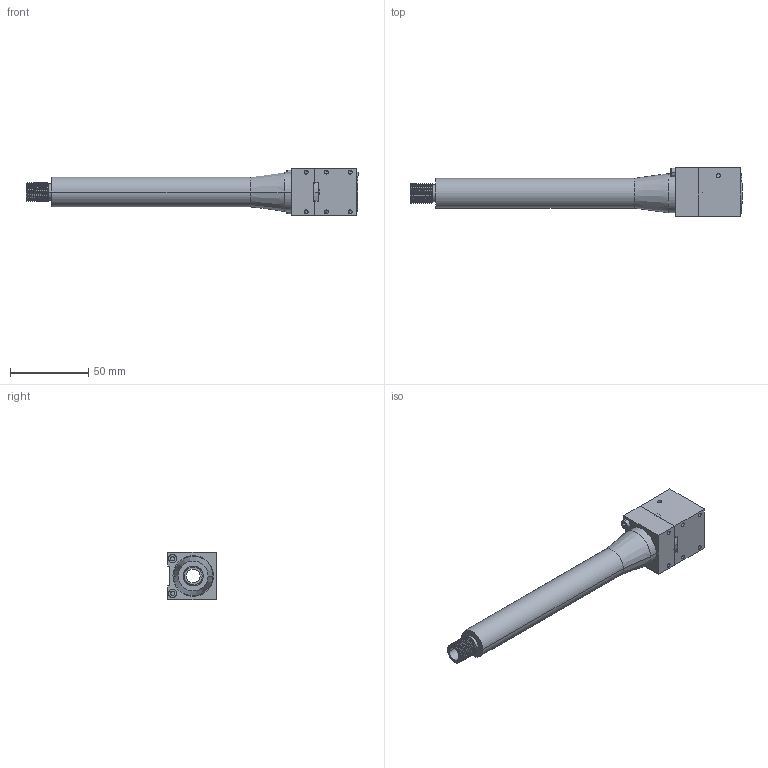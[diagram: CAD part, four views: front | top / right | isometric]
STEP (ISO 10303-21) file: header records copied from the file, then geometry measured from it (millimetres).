
FILE_DESCRIPTION (( 'STEP AP214' ), '1' );
FILE_NAME ('PPDW9 Modcat AR9 barrel and block.STEP', '2020-12-29T19:37:16', ( '' ), ( '' ), 'SwSTEP 2.0', 'SolidWorks 2020', '' );
FILE_SCHEMA (( 'AUTOMOTIVE_DESIGN' ));
Length unit declared in the file: inch
Products named in the file (5): PPDW9 Modcat AR9 barrel and block; PPDW9 Modcat AR9 barrel block clamp; PPDW9 Modcat AR9 barrel block; Barrel AR9 9x19 ; M3 x 25mm SHCS 91290A125_BLACK_91290A125
Assembly tree (5 placements, depth 2):
  PPDW9 Modcat AR9 barrel and block
    PPDW9 Modcat AR9 barrel block
    PPDW9 Modcat AR9 barrel block clamp
    M3 x 25mm SHCS 91290A125_BLACK_91290A125  x2
    Barrel AR9 9x19 
Bounding box: 212.14 x 31.25 x 30.48 mm (x, y, z)
Volume: 73259.7 mm3; surface area: 33060.2 mm2
Topology: 5 solids, 5 shells, 577 faces, 1595 edges, 1046 vertices
Faces by surface type: cylinder 375, plane 118, cone 47, bspline 35, torus 2
Entity records: 23994 total; most frequent: CARTESIAN_POINT 14516, ORIENTED_EDGE 2184, DIRECTION 1522, EDGE_CURVE 1092, VERTEX_POINT 720, AXIS2_PLACEMENT_3D 516, LINE 490, VECTOR 490
